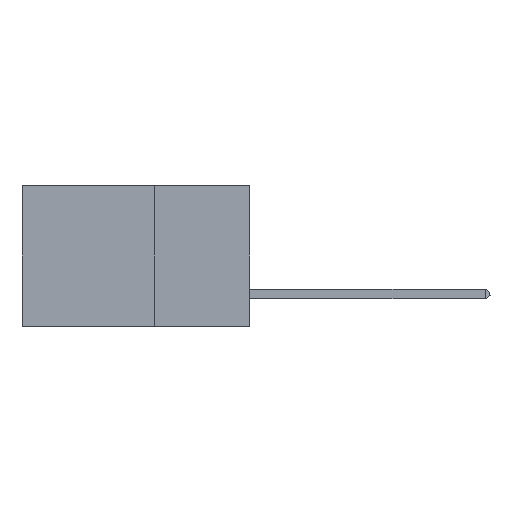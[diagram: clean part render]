
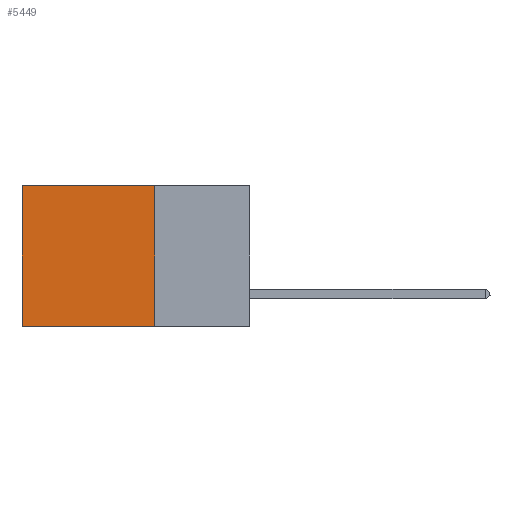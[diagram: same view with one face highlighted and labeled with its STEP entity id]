
A CAD part, left-side view. The second image highlights one B-rep face of the part: STEP entity #5449.
In plain terms, the highlighted planar face has unit normal (-1, 0, 0).
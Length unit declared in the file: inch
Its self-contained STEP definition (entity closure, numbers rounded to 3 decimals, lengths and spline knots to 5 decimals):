
#247 = LINE ( 'NONE', #20363, #8322 ) ;
#344 = VECTOR ( 'NONE', #6349, 39.37008 ) ;
#543 = EDGE_CURVE ( 'NONE', #19498, #16210, #18845, .T. ) ;
#603 = DIRECTION ( 'NONE',  ( 1., 0., 0. ) ) ;
#611 = ORIENTED_EDGE ( 'NONE', *, *, #10803, .T. ) ;
#1620 = CARTESIAN_POINT ( 'NONE',  ( 0.2875, 0.6, 0. ) ) ;
#2579 = EDGE_CURVE ( 'NONE', #7920, #16210, #247, .T. ) ;
#3857 = AXIS2_PLACEMENT_3D ( 'NONE', #4028, #603, #15184 ) ;
#4028 = CARTESIAN_POINT ( 'NONE',  ( 0.2875, 0.25, 0. ) ) ;
#4643 = ORIENTED_EDGE ( 'NONE', *, *, #13337, .F. ) ;
#4956 = FACE_OUTER_BOUND ( 'NONE', #20296, .T. ) ;
#4984 = CARTESIAN_POINT ( 'NONE',  ( 0.2875, 0.25, 0. ) ) ;
#5449 = ADVANCED_FACE ( 'NONE', ( #4956 ), #13453, .F. ) ;
#6349 = DIRECTION ( 'NONE',  ( 0., 0., -1. ) ) ;
#6350 = CARTESIAN_POINT ( 'NONE',  ( 0.2875, 0.25, -0.37 ) ) ;
#7621 = DIRECTION ( 'NONE',  ( 0., 0., -1. ) ) ;
#7920 = VERTEX_POINT ( 'NONE', #6350 ) ;
#8322 = VECTOR ( 'NONE', #13905, 39.37008 ) ;
#8719 = CARTESIAN_POINT ( 'NONE',  ( 0.2875, 0.6, -0.37 ) ) ;
#9893 = ORIENTED_EDGE ( 'NONE', *, *, #543, .T. ) ;
#10134 = VECTOR ( 'NONE', #7621, 39.37008 ) ;
#10731 = VECTOR ( 'NONE', #19888, 39.37008 ) ;
#10803 = EDGE_CURVE ( 'NONE', #11627, #19498, #14451, .T. ) ;
#11627 = VERTEX_POINT ( 'NONE', #4984 ) ;
#13074 = CARTESIAN_POINT ( 'NONE',  ( 0.2875, 0.6, 0. ) ) ;
#13337 = EDGE_CURVE ( 'NONE', #11627, #7920, #19817, .T. ) ;
#13453 = PLANE ( 'NONE',  #3857 ) ;
#13905 = DIRECTION ( 'NONE',  ( 0., 1., 0. ) ) ;
#14451 = LINE ( 'NONE', #14812, #10731 ) ;
#14812 = CARTESIAN_POINT ( 'NONE',  ( 0.2875, 0.25, 0. ) ) ;
#15184 = DIRECTION ( 'NONE',  ( 0., 0., -1. ) ) ;
#16210 = VERTEX_POINT ( 'NONE', #8719 ) ;
#16513 = ORIENTED_EDGE ( 'NONE', *, *, #2579, .F. ) ;
#17109 = CARTESIAN_POINT ( 'NONE',  ( 0.2875, 0.25, 0. ) ) ;
#18845 = LINE ( 'NONE', #1620, #344 ) ;
#19498 = VERTEX_POINT ( 'NONE', #13074 ) ;
#19817 = LINE ( 'NONE', #17109, #10134 ) ;
#19888 = DIRECTION ( 'NONE',  ( 0., 1., 0. ) ) ;
#20296 = EDGE_LOOP ( 'NONE', ( #9893, #16513, #4643, #611 ) ) ;
#20363 = CARTESIAN_POINT ( 'NONE',  ( 0.2875, 0.25, -0.37 ) ) ;
